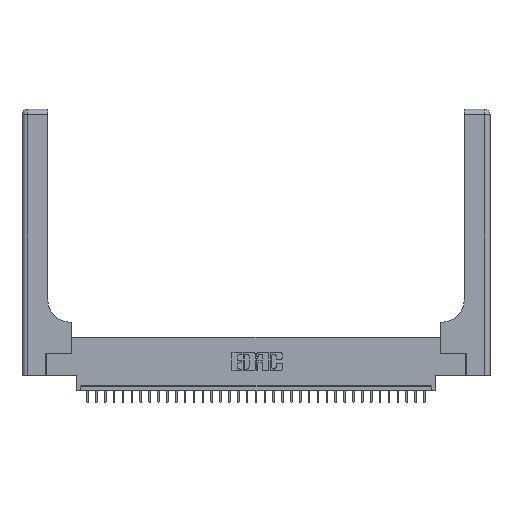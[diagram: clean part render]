
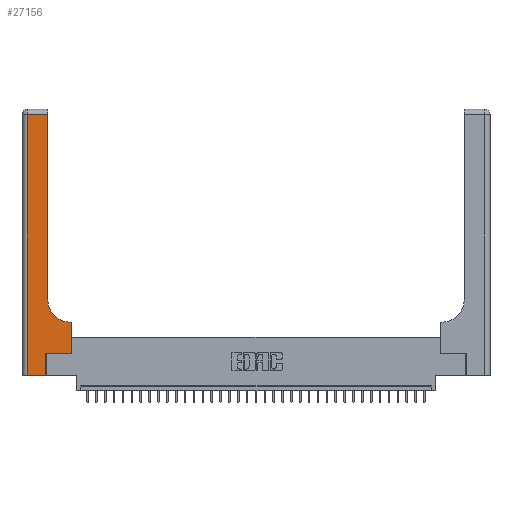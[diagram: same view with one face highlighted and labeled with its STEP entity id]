
A CAD part, top view. The second image highlights one B-rep face of the part: STEP entity #27156.
In plain terms, the highlighted planar face has unit normal (0, 0, 1).
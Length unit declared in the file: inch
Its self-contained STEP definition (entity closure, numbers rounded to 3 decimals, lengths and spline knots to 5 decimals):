
#135 = DIRECTION ( 'NONE',  ( -1., 0., 0. ) ) ;
#1174 = CARTESIAN_POINT ( 'NONE',  ( 0.06, 3., 0.37 ) ) ;
#1224 = EDGE_CURVE ( 'NONE', #6285, #18032, #17695, .T. ) ;
#1302 = PLANE ( 'NONE',  #27366 ) ;
#2179 = ORIENTED_EDGE ( 'NONE', *, *, #19160, .T. ) ;
#3626 = VECTOR ( 'NONE', #135, 39.37008 ) ;
#6285 = VERTEX_POINT ( 'NONE', #33054 ) ;
#6996 = DIRECTION ( 'NONE',  ( 0., 1., 0. ) ) ;
#7239 = EDGE_CURVE ( 'NONE', #18013, #31293, #14968, .T. ) ;
#7704 = DIRECTION ( 'NONE',  ( 1., 0., 0. ) ) ;
#7979 = CARTESIAN_POINT ( 'NONE',  ( 0.2915, 3., 0.37 ) ) ;
#8102 = VECTOR ( 'NONE', #22182, 39.37008 ) ;
#8471 = ORIENTED_EDGE ( 'NONE', *, *, #31526, .T. ) ;
#8492 = CARTESIAN_POINT ( 'NONE',  ( 0.06, 0., 0.37 ) ) ;
#8984 = CARTESIAN_POINT ( 'NONE',  ( 0.2915, 2.94, 0.37 ) ) ;
#9009 = EDGE_CURVE ( 'NONE', #31293, #10666, #34461, .T. ) ;
#9145 = DIRECTION ( 'NONE',  ( -1., 0., 0. ) ) ;
#9283 = DIRECTION ( 'NONE',  ( 0., 1., 0. ) ) ;
#9834 = CARTESIAN_POINT ( 'NONE',  ( 0.2915, 0.85, 0.37 ) ) ;
#9994 = ORIENTED_EDGE ( 'NONE', *, *, #12620, .T. ) ;
#10117 = CARTESIAN_POINT ( 'NONE',  ( 0.269, 0.25, 0.37 ) ) ;
#10493 = DIRECTION ( 'NONE',  ( 0., 0., -1. ) ) ;
#10666 = VERTEX_POINT ( 'NONE', #10949 ) ;
#10949 = CARTESIAN_POINT ( 'NONE',  ( 0.5585, 0.25, 0.37 ) ) ;
#11055 = CARTESIAN_POINT ( 'NONE',  ( 0.5585, 0.6, 0.37 ) ) ;
#12311 = CARTESIAN_POINT ( 'NONE',  ( 0.269, 0., 0.37 ) ) ;
#12620 = EDGE_CURVE ( 'NONE', #10666, #32737, #18015, .T. ) ;
#12866 = VECTOR ( 'NONE', #9283, 39.37008 ) ;
#13663 = ORIENTED_EDGE ( 'NONE', *, *, #32461, .T. ) ;
#14662 = DIRECTION ( 'NONE',  ( 0., 0., -1. ) ) ;
#14711 = LINE ( 'NONE', #1174, #21865 ) ;
#14960 = CARTESIAN_POINT ( 'NONE',  ( 0., 2.94, 0.37 ) ) ;
#14968 = LINE ( 'NONE', #12311, #12866 ) ;
#15260 = VECTOR ( 'NONE', #6996, 39.37008 ) ;
#15299 = LINE ( 'NONE', #32504, #3626 ) ;
#15693 = CARTESIAN_POINT ( 'NONE',  ( 0.269, 0.25, 0.37 ) ) ;
#15726 = VECTOR ( 'NONE', #7704, 39.37008 ) ;
#16045 = LINE ( 'NONE', #24403, #15726 ) ;
#17065 = VECTOR ( 'NONE', #20946, 39.37008 ) ;
#17673 = CARTESIAN_POINT ( 'NONE',  ( 0., 3., 0.37 ) ) ;
#17695 = CIRCLE ( 'NONE', #21072, 0.25 ) ;
#18013 = VERTEX_POINT ( 'NONE', #20501 ) ;
#18015 = LINE ( 'NONE', #31353, #15260 ) ;
#18032 = VERTEX_POINT ( 'NONE', #9834 ) ;
#18196 = ORIENTED_EDGE ( 'NONE', *, *, #25636, .T. ) ;
#18975 = VECTOR ( 'NONE', #27948, 39.37008 ) ;
#19160 = EDGE_CURVE ( 'NONE', #18032, #28186, #26832, .T. ) ;
#20305 = EDGE_CURVE ( 'NONE', #32737, #6285, #15299, .T. ) ;
#20470 = LINE ( 'NONE', #14960, #18975 ) ;
#20501 = CARTESIAN_POINT ( 'NONE',  ( 0.269, 0., 0.37 ) ) ;
#20946 = DIRECTION ( 'NONE',  ( 1., 0., 0. ) ) ;
#21072 = AXIS2_PLACEMENT_3D ( 'NONE', #34838, #10493, #24526 ) ;
#21810 = ORIENTED_EDGE ( 'NONE', *, *, #7239, .T. ) ;
#21865 = VECTOR ( 'NONE', #30352, 39.37008 ) ;
#22182 = DIRECTION ( 'NONE',  ( 0., 1., 0. ) ) ;
#23373 = ORIENTED_EDGE ( 'NONE', *, *, #1224, .T. ) ;
#23655 = EDGE_LOOP ( 'NONE', ( #2179, #8471, #13663, #18196, #21810, #26986, #9994, #31110, #23373 ) ) ;
#24403 = CARTESIAN_POINT ( 'NONE',  ( 0., 0., 0.37 ) ) ;
#24526 = DIRECTION ( 'NONE',  ( 1., 0., 0. ) ) ;
#24941 = CARTESIAN_POINT ( 'NONE',  ( 0.06, 2.94, 0.37 ) ) ;
#25636 = EDGE_CURVE ( 'NONE', #32334, #18013, #16045, .T. ) ;
#26832 = LINE ( 'NONE', #7979, #8102 ) ;
#26986 = ORIENTED_EDGE ( 'NONE', *, *, #9009, .T. ) ;
#27156 = ADVANCED_FACE ( 'NONE', ( #30828 ), #1302, .F. ) ;
#27366 = AXIS2_PLACEMENT_3D ( 'NONE', #17673, #14662, #9145 ) ;
#27948 = DIRECTION ( 'NONE',  ( -1., 0., 0. ) ) ;
#28186 = VERTEX_POINT ( 'NONE', #8984 ) ;
#30352 = DIRECTION ( 'NONE',  ( 0., -1., 0. ) ) ;
#30828 = FACE_OUTER_BOUND ( 'NONE', #23655, .T. ) ;
#31110 = ORIENTED_EDGE ( 'NONE', *, *, #20305, .T. ) ;
#31293 = VERTEX_POINT ( 'NONE', #15693 ) ;
#31353 = CARTESIAN_POINT ( 'NONE',  ( 0.5585, 0.25, 0.37 ) ) ;
#31526 = EDGE_CURVE ( 'NONE', #28186, #34855, #20470, .T. ) ;
#32334 = VERTEX_POINT ( 'NONE', #8492 ) ;
#32461 = EDGE_CURVE ( 'NONE', #34855, #32334, #14711, .T. ) ;
#32504 = CARTESIAN_POINT ( 'NONE',  ( 0.2915, 0.6, 0.37 ) ) ;
#32737 = VERTEX_POINT ( 'NONE', #11055 ) ;
#33054 = CARTESIAN_POINT ( 'NONE',  ( 0.5415, 0.6, 0.37 ) ) ;
#34461 = LINE ( 'NONE', #10117, #17065 ) ;
#34838 = CARTESIAN_POINT ( 'NONE',  ( 0.5415, 0.85, 0.37 ) ) ;
#34855 = VERTEX_POINT ( 'NONE', #24941 ) ;
